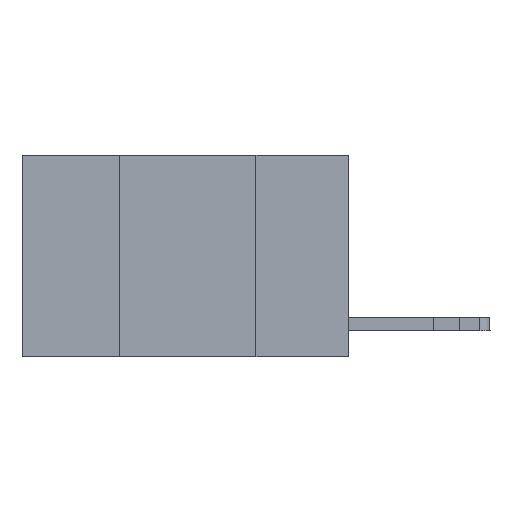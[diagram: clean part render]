
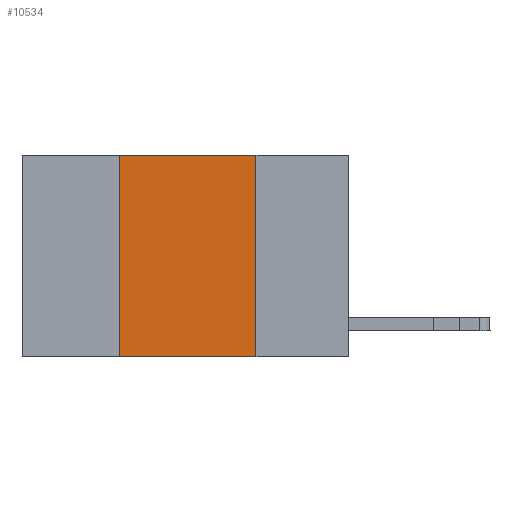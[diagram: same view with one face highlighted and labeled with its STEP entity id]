
A CAD part, left-side view. The second image highlights one B-rep face of the part: STEP entity #10534.
In plain terms, the highlighted planar face has unit normal (-1, 0, 0).
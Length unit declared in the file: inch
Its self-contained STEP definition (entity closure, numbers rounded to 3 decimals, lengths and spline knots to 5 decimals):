
#112 = AXIS2_PLACEMENT_3D ( 'NONE', #19386, #17678, #12250 ) ;
#1625 = VERTEX_POINT ( 'NONE', #12674 ) ;
#2056 = LINE ( 'NONE', #19014, #11299 ) ;
#2415 = ORIENTED_EDGE ( 'NONE', *, *, #11172, .F. ) ;
#3353 = DIRECTION ( 'NONE',  ( 0., -1., 0. ) ) ;
#3834 = CARTESIAN_POINT ( 'NONE',  ( 0., 0.17, -0.37 ) ) ;
#4326 = DIRECTION ( 'NONE',  ( 0., 0., 1. ) ) ;
#4442 = LINE ( 'NONE', #7738, #7822 ) ;
#5103 = VERTEX_POINT ( 'NONE', #3834 ) ;
#5553 = FACE_OUTER_BOUND ( 'NONE', #18470, .T. ) ;
#6626 = VECTOR ( 'NONE', #10111, 39.37008 ) ;
#6849 = ORIENTED_EDGE ( 'NONE', *, *, #19600, .T. ) ;
#6954 = DIRECTION ( 'NONE',  ( 0., 0., -1. ) ) ;
#7632 = EDGE_CURVE ( 'NONE', #1625, #10107, #2056, .T. ) ;
#7738 = CARTESIAN_POINT ( 'NONE',  ( 0., 0.42, 0. ) ) ;
#7822 = VECTOR ( 'NONE', #4326, 39.37008 ) ;
#9663 = CARTESIAN_POINT ( 'NONE',  ( 0., 0.42, -0.37 ) ) ;
#9825 = VERTEX_POINT ( 'NONE', #9663 ) ;
#10107 = VERTEX_POINT ( 'NONE', #11036 ) ;
#10111 = DIRECTION ( 'NONE',  ( 0., -1., 0. ) ) ;
#10212 = VECTOR ( 'NONE', #6954, 39.37008 ) ;
#10375 = CARTESIAN_POINT ( 'NONE',  ( 0., 0.17, 0. ) ) ;
#10534 = ADVANCED_FACE ( 'NONE', ( #5553 ), #16180, .F. ) ;
#11036 = CARTESIAN_POINT ( 'NONE',  ( 0., 0.17, 0. ) ) ;
#11172 = EDGE_CURVE ( 'NONE', #9825, #1625, #4442, .T. ) ;
#11299 = VECTOR ( 'NONE', #3353, 39.37008 ) ;
#12250 = DIRECTION ( 'NONE',  ( 0., 0., -1. ) ) ;
#12674 = CARTESIAN_POINT ( 'NONE',  ( 0., 0.42, 0. ) ) ;
#15987 = EDGE_CURVE ( 'NONE', #10107, #5103, #21010, .T. ) ;
#16180 = PLANE ( 'NONE',  #112 ) ;
#16581 = ORIENTED_EDGE ( 'NONE', *, *, #15987, .F. ) ;
#16887 = LINE ( 'NONE', #18706, #6626 ) ;
#17678 = DIRECTION ( 'NONE',  ( 1., 0., 0. ) ) ;
#18470 = EDGE_LOOP ( 'NONE', ( #16581, #22237, #2415, #6849 ) ) ;
#18706 = CARTESIAN_POINT ( 'NONE',  ( 0., 0.6, -0.37 ) ) ;
#19014 = CARTESIAN_POINT ( 'NONE',  ( 0., 0.6, 0. ) ) ;
#19386 = CARTESIAN_POINT ( 'NONE',  ( 0., 0.6, 0. ) ) ;
#19600 = EDGE_CURVE ( 'NONE', #9825, #5103, #16887, .T. ) ;
#21010 = LINE ( 'NONE', #10375, #10212 ) ;
#22237 = ORIENTED_EDGE ( 'NONE', *, *, #7632, .F. ) ;
